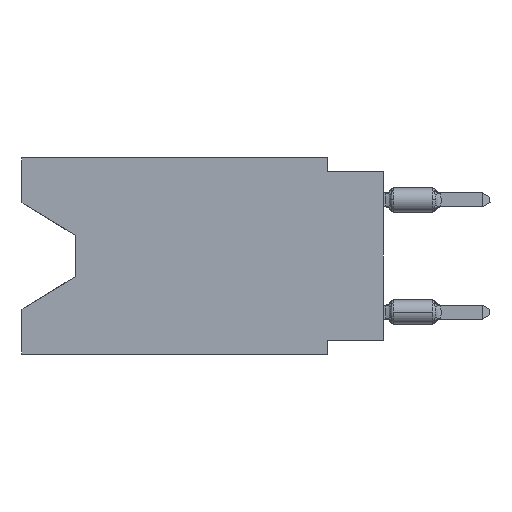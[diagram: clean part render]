
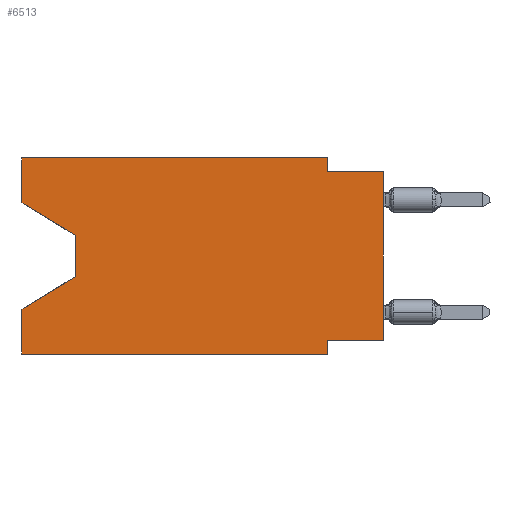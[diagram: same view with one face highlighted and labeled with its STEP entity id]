
A CAD part, left-side view. The second image highlights one B-rep face of the part: STEP entity #6513.
In plain terms, the highlighted planar face has unit normal (-1, 0, 0).
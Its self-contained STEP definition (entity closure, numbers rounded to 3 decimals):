
#123 = VECTOR ( 'NONE', #30603, 1000. ) ;
#624 = EDGE_CURVE ( 'NONE', #10181, #24088, #9135, .T. ) ;
#1046 = CARTESIAN_POINT ( 'NONE',  ( 0., 16.383, 0. ) ) ;
#1078 = VERTEX_POINT ( 'NONE', #2389 ) ;
#2102 = LINE ( 'NONE', #19220, #16957 ) ;
#2389 = CARTESIAN_POINT ( 'NONE',  ( 0., 13.97, -5.385 ) ) ;
#2852 = VERTEX_POINT ( 'NONE', #28207 ) ;
#2930 = ORIENTED_EDGE ( 'NONE', *, *, #12816, .T. ) ;
#3364 = LINE ( 'NONE', #27164, #24827 ) ;
#4204 = LINE ( 'NONE', #18799, #5260 ) ;
#4459 = CARTESIAN_POINT ( 'NONE',  ( 0., 16.383, 0. ) ) ;
#4661 = EDGE_CURVE ( 'NONE', #2852, #10117, #14700, .T. ) ;
#4971 = ORIENTED_EDGE ( 'NONE', *, *, #14619, .F. ) ;
#5260 = VECTOR ( 'NONE', #21497, 1000. ) ;
#5991 = VERTEX_POINT ( 'NONE', #1046 ) ;
#6374 = AXIS2_PLACEMENT_3D ( 'NONE', #24951, #10840, #13078 ) ;
#6513 = ADVANCED_FACE ( 'NONE', ( #15448 ), #25109, .F. ) ;
#7471 = EDGE_CURVE ( 'NONE', #1078, #24088, #17345, .T. ) ;
#7646 = CARTESIAN_POINT ( 'NONE',  ( 0., 16.383, -8.89 ) ) ;
#8407 = VECTOR ( 'NONE', #15805, 1000. ) ;
#8636 = DIRECTION ( 'NONE',  ( 0., -1., 0. ) ) ;
#8758 = CARTESIAN_POINT ( 'NONE',  ( 0., 13.97, -3.505 ) ) ;
#9135 = LINE ( 'NONE', #18452, #19286 ) ;
#9351 = VERTEX_POINT ( 'NONE', #8758 ) ;
#9640 = EDGE_CURVE ( 'NONE', #5991, #14935, #28662, .T. ) ;
#9891 = CARTESIAN_POINT ( 'NONE',  ( 0., 16.383, -6.852 ) ) ;
#9979 = EDGE_CURVE ( 'NONE', #2852, #14733, #2102, .T. ) ;
#10092 = CARTESIAN_POINT ( 'NONE',  ( 0., 0., -8.255 ) ) ;
#10117 = VERTEX_POINT ( 'NONE', #29497 ) ;
#10181 = VERTEX_POINT ( 'NONE', #7646 ) ;
#10244 = DIRECTION ( 'NONE',  ( 0., 1., 0. ) ) ;
#10539 = LINE ( 'NONE', #12765, #17472 ) ;
#10840 = DIRECTION ( 'NONE',  ( 1., 0., 0. ) ) ;
#10911 = ORIENTED_EDGE ( 'NONE', *, *, #9640, .F. ) ;
#11269 = ORIENTED_EDGE ( 'NONE', *, *, #22667, .F. ) ;
#11308 = ORIENTED_EDGE ( 'NONE', *, *, #7471, .T. ) ;
#12450 = VERTEX_POINT ( 'NONE', #13132 ) ;
#12765 = CARTESIAN_POINT ( 'NONE',  ( 0., 16.383, -2.038 ) ) ;
#12787 = EDGE_CURVE ( 'NONE', #21744, #9351, #10539, .T. ) ;
#12816 = EDGE_CURVE ( 'NONE', #10181, #24706, #20201, .T. ) ;
#12845 = ORIENTED_EDGE ( 'NONE', *, *, #12787, .T. ) ;
#13078 = DIRECTION ( 'NONE',  ( 0., 0., -1. ) ) ;
#13132 = CARTESIAN_POINT ( 'NONE',  ( 0., 2.54, -0.635 ) ) ;
#13615 = ORIENTED_EDGE ( 'NONE', *, *, #26535, .F. ) ;
#14608 = ORIENTED_EDGE ( 'NONE', *, *, #9979, .T. ) ;
#14619 = EDGE_CURVE ( 'NONE', #10117, #24706, #20124, .T. ) ;
#14680 = CARTESIAN_POINT ( 'NONE',  ( 0., 13.97, -5.385 ) ) ;
#14700 = LINE ( 'NONE', #10092, #14902 ) ;
#14733 = VERTEX_POINT ( 'NONE', #30882 ) ;
#14902 = VECTOR ( 'NONE', #10244, 1000. ) ;
#14935 = VERTEX_POINT ( 'NONE', #27219 ) ;
#15448 = FACE_OUTER_BOUND ( 'NONE', #20851, .T. ) ;
#15805 = DIRECTION ( 'NONE',  ( 0., -1., 0. ) ) ;
#16811 = ORIENTED_EDGE ( 'NONE', *, *, #624, .F. ) ;
#16957 = VECTOR ( 'NONE', #21771, 1000. ) ;
#17345 = LINE ( 'NONE', #14680, #28696 ) ;
#17412 = EDGE_CURVE ( 'NONE', #9351, #1078, #4204, .T. ) ;
#17472 = VECTOR ( 'NONE', #30333, 1000. ) ;
#18051 = DIRECTION ( 'NONE',  ( 0., 0., -1. ) ) ;
#18452 = CARTESIAN_POINT ( 'NONE',  ( 0., 16.383, 0. ) ) ;
#18472 = CARTESIAN_POINT ( 'NONE',  ( 0., 0., -0.635 ) ) ;
#18751 = EDGE_CURVE ( 'NONE', #21744, #5991, #20627, .T. ) ;
#18799 = CARTESIAN_POINT ( 'NONE',  ( 0., 13.97, -3.505 ) ) ;
#19220 = CARTESIAN_POINT ( 'NONE',  ( 0., 0., 0. ) ) ;
#19286 = VECTOR ( 'NONE', #28131, 1000. ) ;
#20124 = LINE ( 'NONE', #24874, #20616 ) ;
#20201 = LINE ( 'NONE', #25435, #30115 ) ;
#20616 = VECTOR ( 'NONE', #18051, 1000. ) ;
#20627 = LINE ( 'NONE', #4459, #123 ) ;
#20851 = EDGE_LOOP ( 'NONE', ( #12845, #28220, #11308, #16811, #2930, #4971, #25609, #14608, #11269, #13615, #10911, #29889 ) ) ;
#21207 = CARTESIAN_POINT ( 'NONE',  ( 0., 2.54, -8.89 ) ) ;
#21384 = CARTESIAN_POINT ( 'NONE',  ( 0., 16.383, 0. ) ) ;
#21497 = DIRECTION ( 'NONE',  ( 0., 0., -1. ) ) ;
#21744 = VERTEX_POINT ( 'NONE', #23058 ) ;
#21771 = DIRECTION ( 'NONE',  ( 0., 0., 1. ) ) ;
#22667 = EDGE_CURVE ( 'NONE', #12450, #14733, #23105, .T. ) ;
#23058 = CARTESIAN_POINT ( 'NONE',  ( 0., 16.383, -2.038 ) ) ;
#23105 = LINE ( 'NONE', #18472, #8407 ) ;
#23554 = VECTOR ( 'NONE', #25987, 1000. ) ;
#24088 = VERTEX_POINT ( 'NONE', #9891 ) ;
#24706 = VERTEX_POINT ( 'NONE', #21207 ) ;
#24827 = VECTOR ( 'NONE', #25098, 1000. ) ;
#24874 = CARTESIAN_POINT ( 'NONE',  ( 0., 2.54, -8.89 ) ) ;
#24951 = CARTESIAN_POINT ( 'NONE',  ( 0., 16.383, 0. ) ) ;
#25098 = DIRECTION ( 'NONE',  ( 0., 0., -1. ) ) ;
#25109 = PLANE ( 'NONE',  #6374 ) ;
#25435 = CARTESIAN_POINT ( 'NONE',  ( 0., 16.383, -8.89 ) ) ;
#25609 = ORIENTED_EDGE ( 'NONE', *, *, #4661, .F. ) ;
#25987 = DIRECTION ( 'NONE',  ( 0., -1., 0. ) ) ;
#26535 = EDGE_CURVE ( 'NONE', #14935, #12450, #3364, .T. ) ;
#26725 = DIRECTION ( 'NONE',  ( 0., 0.855, -0.519 ) ) ;
#27164 = CARTESIAN_POINT ( 'NONE',  ( 0., 2.54, 0. ) ) ;
#27219 = CARTESIAN_POINT ( 'NONE',  ( 0., 2.54, 0. ) ) ;
#28131 = DIRECTION ( 'NONE',  ( 0., 0., 1. ) ) ;
#28207 = CARTESIAN_POINT ( 'NONE',  ( 0., 0., -8.255 ) ) ;
#28220 = ORIENTED_EDGE ( 'NONE', *, *, #17412, .T. ) ;
#28662 = LINE ( 'NONE', #21384, #23554 ) ;
#28696 = VECTOR ( 'NONE', #26725, 1000. ) ;
#29497 = CARTESIAN_POINT ( 'NONE',  ( 0., 2.54, -8.255 ) ) ;
#29889 = ORIENTED_EDGE ( 'NONE', *, *, #18751, .F. ) ;
#30115 = VECTOR ( 'NONE', #8636, 1000. ) ;
#30333 = DIRECTION ( 'NONE',  ( 0., -0.855, -0.519 ) ) ;
#30603 = DIRECTION ( 'NONE',  ( 0., 0., 1. ) ) ;
#30882 = CARTESIAN_POINT ( 'NONE',  ( 0., 0., -0.635 ) ) ;
